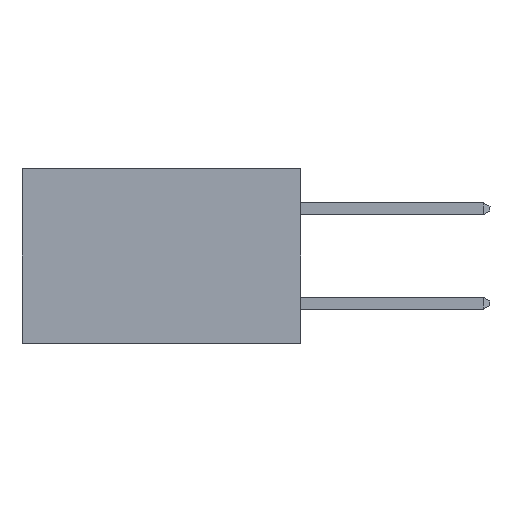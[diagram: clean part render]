
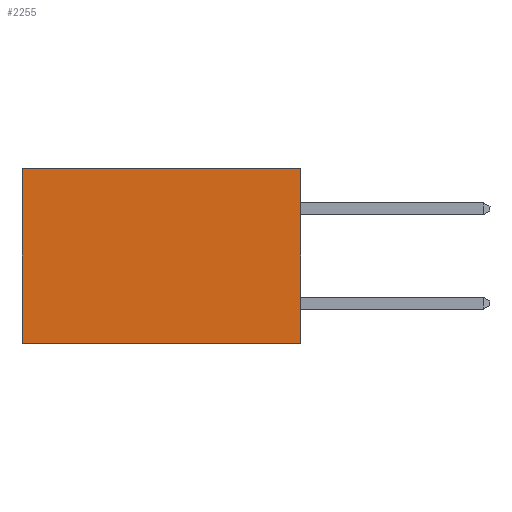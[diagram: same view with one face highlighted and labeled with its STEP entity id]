
A CAD part, left-side view. The second image highlights one B-rep face of the part: STEP entity #2255.
In plain terms, the highlighted planar face has unit normal (-1, 0, 0).
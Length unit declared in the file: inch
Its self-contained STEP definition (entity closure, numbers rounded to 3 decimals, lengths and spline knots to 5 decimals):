
#104 = VERTEX_POINT ( 'NONE', #1213 ) ;
#889 = EDGE_LOOP ( 'NONE', ( #9303, #7836, #5789, #5579 ) ) ;
#966 = VECTOR ( 'NONE', #4423, 39.37008 ) ;
#991 = VERTEX_POINT ( 'NONE', #6703 ) ;
#1213 = CARTESIAN_POINT ( 'NONE',  ( 0.277, 0.59, -0.37 ) ) ;
#1772 = VERTEX_POINT ( 'NONE', #7282 ) ;
#1905 = VERTEX_POINT ( 'NONE', #3774 ) ;
#2255 = ADVANCED_FACE ( 'NONE', ( #2283 ), #3422, .F. ) ;
#2283 = FACE_OUTER_BOUND ( 'NONE', #889, .T. ) ;
#2535 = CARTESIAN_POINT ( 'NONE',  ( 0.277, 0.59, -0.37 ) ) ;
#2550 = DIRECTION ( 'NONE',  ( 0., 0., -1. ) ) ;
#3065 = LINE ( 'NONE', #2535, #5497 ) ;
#3422 = PLANE ( 'NONE',  #5853 ) ;
#3640 = CARTESIAN_POINT ( 'NONE',  ( 0.277, 0., -0.37 ) ) ;
#3774 = CARTESIAN_POINT ( 'NONE',  ( 0.277, 0., -0.37 ) ) ;
#4195 = CARTESIAN_POINT ( 'NONE',  ( 0.277, 0., -0.37 ) ) ;
#4269 = EDGE_CURVE ( 'NONE', #1772, #991, #6608, .T. ) ;
#4423 = DIRECTION ( 'NONE',  ( 0., 0., -1. ) ) ;
#4450 = EDGE_CURVE ( 'NONE', #1772, #1905, #8718, .T. ) ;
#4605 = EDGE_CURVE ( 'NONE', #1905, #104, #7335, .T. ) ;
#5235 = DIRECTION ( 'NONE',  ( 0., 0., -1. ) ) ;
#5266 = DIRECTION ( 'NONE',  ( 1., 0., 0. ) ) ;
#5497 = VECTOR ( 'NONE', #2550, 39.37008 ) ;
#5517 = VECTOR ( 'NONE', #9660, 39.37008 ) ;
#5579 = ORIENTED_EDGE ( 'NONE', *, *, #4269, .T. ) ;
#5789 = ORIENTED_EDGE ( 'NONE', *, *, #4450, .F. ) ;
#5853 = AXIS2_PLACEMENT_3D ( 'NONE', #3640, #5266, #5235 ) ;
#6608 = LINE ( 'NONE', #7088, #8614 ) ;
#6703 = CARTESIAN_POINT ( 'NONE',  ( 0.277, 0.59, 0. ) ) ;
#7080 = DIRECTION ( 'NONE',  ( 0., 1., 0. ) ) ;
#7088 = CARTESIAN_POINT ( 'NONE',  ( 0.277, 0., 0. ) ) ;
#7282 = CARTESIAN_POINT ( 'NONE',  ( 0.277, 0., 0. ) ) ;
#7335 = LINE ( 'NONE', #7455, #5517 ) ;
#7455 = CARTESIAN_POINT ( 'NONE',  ( 0.277, 0., -0.37 ) ) ;
#7836 = ORIENTED_EDGE ( 'NONE', *, *, #4605, .F. ) ;
#8430 = EDGE_CURVE ( 'NONE', #991, #104, #3065, .T. ) ;
#8614 = VECTOR ( 'NONE', #7080, 39.37008 ) ;
#8718 = LINE ( 'NONE', #4195, #966 ) ;
#9303 = ORIENTED_EDGE ( 'NONE', *, *, #8430, .T. ) ;
#9660 = DIRECTION ( 'NONE',  ( 0., 1., 0. ) ) ;
